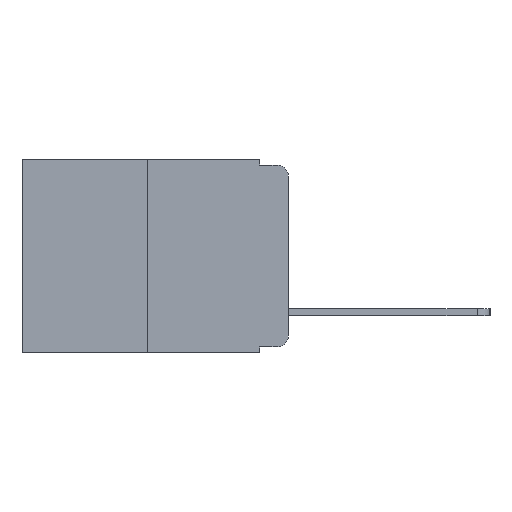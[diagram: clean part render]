
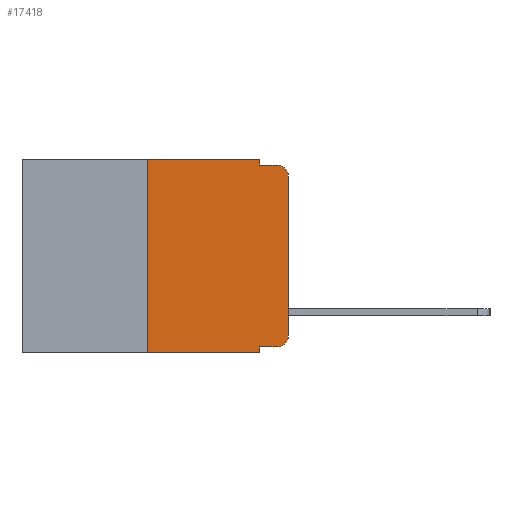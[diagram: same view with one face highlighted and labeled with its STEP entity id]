
A CAD part, left-side view. The second image highlights one B-rep face of the part: STEP entity #17418.
In plain terms, the highlighted planar face has unit normal (-1, 0, 0).
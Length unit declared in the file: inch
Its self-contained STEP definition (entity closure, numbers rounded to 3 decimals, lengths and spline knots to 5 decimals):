
#475 = VECTOR ( 'NONE', #1644, 39.37008 ) ;
#731 = VERTEX_POINT ( 'NONE', #6774 ) ;
#1063 = DIRECTION ( 'NONE',  ( 0., -1., 0. ) ) ;
#1380 = CARTESIAN_POINT ( 'NONE',  ( 0., 0.051, 0. ) ) ;
#1389 = VERTEX_POINT ( 'NONE', #8091 ) ;
#1644 = DIRECTION ( 'NONE',  ( 0., 0., -1. ) ) ;
#1809 = VERTEX_POINT ( 'NONE', #12674 ) ;
#1820 = EDGE_CURVE ( 'NONE', #18503, #8082, #12736, .T. ) ;
#2427 = CARTESIAN_POINT ( 'NONE',  ( 0., 0.02, -0.03 ) ) ;
#2912 = ORIENTED_EDGE ( 'NONE', *, *, #20693, .F. ) ;
#3128 = ORIENTED_EDGE ( 'NONE', *, *, #17628, .F. ) ;
#3530 = ORIENTED_EDGE ( 'NONE', *, *, #15295, .T. ) ;
#4072 = ORIENTED_EDGE ( 'NONE', *, *, #13718, .F. ) ;
#4494 = DIRECTION ( 'NONE',  ( 0., 0., -1. ) ) ;
#4699 = EDGE_CURVE ( 'NONE', #12580, #5796, #4999, .T. ) ;
#4999 = LINE ( 'NONE', #25704, #20338 ) ;
#5796 = VERTEX_POINT ( 'NONE', #16377 ) ;
#5905 = LINE ( 'NONE', #25394, #475 ) ;
#6330 = LINE ( 'NONE', #1380, #21586 ) ;
#6567 = VERTEX_POINT ( 'NONE', #13195 ) ;
#6774 = CARTESIAN_POINT ( 'NONE',  ( 0., 0.051, -0.333 ) ) ;
#6917 = ORIENTED_EDGE ( 'NONE', *, *, #20060, .T. ) ;
#7049 = DIRECTION ( 'NONE',  ( 0., -1., 0. ) ) ;
#7104 = VECTOR ( 'NONE', #14932, 39.37008 ) ;
#7190 = PLANE ( 'NONE',  #21042 ) ;
#7241 = CARTESIAN_POINT ( 'NONE',  ( 0., 0.051, -0.01 ) ) ;
#7288 = LINE ( 'NONE', #21067, #17351 ) ;
#7616 = EDGE_CURVE ( 'NONE', #5796, #8082, #15272, .T. ) ;
#7779 = LINE ( 'NONE', #21808, #17834 ) ;
#8057 = AXIS2_PLACEMENT_3D ( 'NONE', #2427, #16565, #4494 ) ;
#8082 = VERTEX_POINT ( 'NONE', #23724 ) ;
#8091 = CARTESIAN_POINT ( 'NONE',  ( 0., 0.25, 0. ) ) ;
#8591 = DIRECTION ( 'NONE',  ( -1., 0., 0. ) ) ;
#8644 = ORIENTED_EDGE ( 'NONE', *, *, #7616, .T. ) ;
#9193 = DIRECTION ( 'NONE',  ( 0., 0., -1. ) ) ;
#9972 = CARTESIAN_POINT ( 'NONE',  ( 0., 0.02, -0.333 ) ) ;
#10629 = FACE_OUTER_BOUND ( 'NONE', #15313, .T. ) ;
#10841 = ORIENTED_EDGE ( 'NONE', *, *, #16664, .F. ) ;
#11545 = EDGE_CURVE ( 'NONE', #15015, #12580, #16106, .T. ) ;
#12479 = LINE ( 'NONE', #18806, #7104 ) ;
#12580 = VERTEX_POINT ( 'NONE', #14309 ) ;
#12674 = CARTESIAN_POINT ( 'NONE',  ( 0., 0.051, -0.343 ) ) ;
#12736 = LINE ( 'NONE', #7241, #22017 ) ;
#13195 = CARTESIAN_POINT ( 'NONE',  ( 0., 0.051, 0. ) ) ;
#13315 = CARTESIAN_POINT ( 'NONE',  ( 0., 0.25, -0.343 ) ) ;
#13718 = EDGE_CURVE ( 'NONE', #1389, #6567, #7779, .T. ) ;
#14309 = CARTESIAN_POINT ( 'NONE',  ( 0., 0., -0.313 ) ) ;
#14606 = ORIENTED_EDGE ( 'NONE', *, *, #11545, .T. ) ;
#14932 = DIRECTION ( 'NONE',  ( 0., -1., 0. ) ) ;
#15015 = VERTEX_POINT ( 'NONE', #9972 ) ;
#15272 = CIRCLE ( 'NONE', #8057, 0.02 ) ;
#15295 = EDGE_CURVE ( 'NONE', #731, #15015, #12479, .T. ) ;
#15313 = EDGE_LOOP ( 'NONE', ( #16277, #8644, #25757, #10841, #4072, #3128, #6917, #2912, #3530, #14606 ) ) ;
#16106 = CIRCLE ( 'NONE', #17686, 0.02 ) ;
#16277 = ORIENTED_EDGE ( 'NONE', *, *, #4699, .T. ) ;
#16377 = CARTESIAN_POINT ( 'NONE',  ( 0., 0., -0.03 ) ) ;
#16565 = DIRECTION ( 'NONE',  ( -1., 0., 0. ) ) ;
#16664 = EDGE_CURVE ( 'NONE', #6567, #18503, #5905, .T. ) ;
#16741 = CARTESIAN_POINT ( 'NONE',  ( 0., 0.051, -0.01 ) ) ;
#17351 = VECTOR ( 'NONE', #1063, 39.37008 ) ;
#17418 = ADVANCED_FACE ( 'NONE', ( #10629 ), #7190, .F. ) ;
#17628 = EDGE_CURVE ( 'NONE', #21834, #1389, #24866, .T. ) ;
#17686 = AXIS2_PLACEMENT_3D ( 'NONE', #20542, #8591, #22523 ) ;
#17834 = VECTOR ( 'NONE', #23791, 39.37008 ) ;
#18503 = VERTEX_POINT ( 'NONE', #16741 ) ;
#18806 = CARTESIAN_POINT ( 'NONE',  ( 0., 0.051, -0.333 ) ) ;
#19649 = VECTOR ( 'NONE', #23717, 39.37008 ) ;
#20060 = EDGE_CURVE ( 'NONE', #21834, #1809, #7288, .T. ) ;
#20338 = VECTOR ( 'NONE', #23775, 39.37008 ) ;
#20542 = CARTESIAN_POINT ( 'NONE',  ( 0., 0.02, -0.313 ) ) ;
#20693 = EDGE_CURVE ( 'NONE', #731, #1809, #6330, .T. ) ;
#21042 = AXIS2_PLACEMENT_3D ( 'NONE', #24996, #21138, #9193 ) ;
#21067 = CARTESIAN_POINT ( 'NONE',  ( 0., 0.473, -0.343 ) ) ;
#21138 = DIRECTION ( 'NONE',  ( 1., 0., 0. ) ) ;
#21384 = DIRECTION ( 'NONE',  ( 0., 0., -1. ) ) ;
#21586 = VECTOR ( 'NONE', #21384, 39.37008 ) ;
#21725 = CARTESIAN_POINT ( 'NONE',  ( 0., 0.25, 0. ) ) ;
#21808 = CARTESIAN_POINT ( 'NONE',  ( 0., 0.473, 0. ) ) ;
#21834 = VERTEX_POINT ( 'NONE', #13315 ) ;
#22017 = VECTOR ( 'NONE', #7049, 39.37008 ) ;
#22523 = DIRECTION ( 'NONE',  ( 0., 0., -1. ) ) ;
#23717 = DIRECTION ( 'NONE',  ( 0., 0., 1. ) ) ;
#23724 = CARTESIAN_POINT ( 'NONE',  ( 0., 0.02, -0.01 ) ) ;
#23775 = DIRECTION ( 'NONE',  ( 0., 0., 1. ) ) ;
#23791 = DIRECTION ( 'NONE',  ( 0., -1., 0. ) ) ;
#24866 = LINE ( 'NONE', #21725, #19649 ) ;
#24996 = CARTESIAN_POINT ( 'NONE',  ( 0., 0.473, 0. ) ) ;
#25394 = CARTESIAN_POINT ( 'NONE',  ( 0., 0.051, 0. ) ) ;
#25704 = CARTESIAN_POINT ( 'NONE',  ( 0., 0., 0. ) ) ;
#25757 = ORIENTED_EDGE ( 'NONE', *, *, #1820, .F. ) ;
